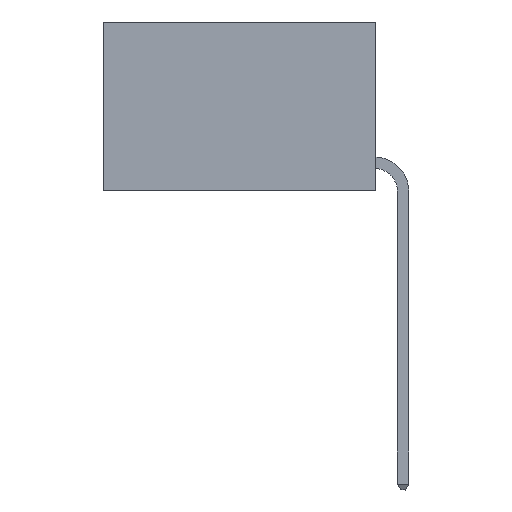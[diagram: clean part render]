
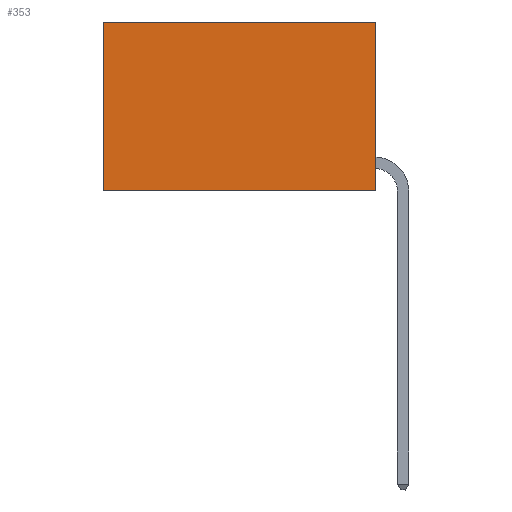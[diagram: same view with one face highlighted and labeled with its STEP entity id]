
A CAD part, left-side view. The second image highlights one B-rep face of the part: STEP entity #353.
In plain terms, the highlighted planar face has unit normal (-1, 0, 0).
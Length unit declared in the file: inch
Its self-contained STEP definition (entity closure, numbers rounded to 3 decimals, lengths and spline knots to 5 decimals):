
#353 = ADVANCED_FACE ( 'NONE', ( #5315 ), #7986, .F. ) ;
#680 = LINE ( 'NONE', #1629, #2735 ) ;
#691 = CARTESIAN_POINT ( 'NONE',  ( 0.2625, 0.6, -0.37 ) ) ;
#824 = VECTOR ( 'NONE', #7838, 39.37008 ) ;
#979 = EDGE_CURVE ( 'NONE', #7030, #5286, #6334, .T. ) ;
#1422 = CARTESIAN_POINT ( 'NONE',  ( 0.2625, 0., -0.37 ) ) ;
#1629 = CARTESIAN_POINT ( 'NONE',  ( 0.2625, 0., 0. ) ) ;
#1760 = EDGE_CURVE ( 'NONE', #7035, #7030, #680, .T. ) ;
#1838 = CARTESIAN_POINT ( 'NONE',  ( 0.2625, 0.6, 0. ) ) ;
#2067 = VECTOR ( 'NONE', #6882, 39.37008 ) ;
#2118 = LINE ( 'NONE', #5071, #8231 ) ;
#2173 = VERTEX_POINT ( 'NONE', #8725 ) ;
#2587 = DIRECTION ( 'NONE',  ( 0., 1., 0. ) ) ;
#2735 = VECTOR ( 'NONE', #2587, 39.37008 ) ;
#2865 = LINE ( 'NONE', #1422, #824 ) ;
#3281 = EDGE_LOOP ( 'NONE', ( #5196, #8546, #10106, #8673 ) ) ;
#3445 = DIRECTION ( 'NONE',  ( 0., 0., -1. ) ) ;
#4118 = EDGE_CURVE ( 'NONE', #7035, #2173, #2118, .T. ) ;
#4558 = CARTESIAN_POINT ( 'NONE',  ( 0.2625, 0., 0. ) ) ;
#5071 = CARTESIAN_POINT ( 'NONE',  ( 0.2625, 0., 0. ) ) ;
#5196 = ORIENTED_EDGE ( 'NONE', *, *, #979, .T. ) ;
#5286 = VERTEX_POINT ( 'NONE', #691 ) ;
#5315 = FACE_OUTER_BOUND ( 'NONE', #3281, .T. ) ;
#5656 = EDGE_CURVE ( 'NONE', #2173, #5286, #2865, .T. ) ;
#6306 = CARTESIAN_POINT ( 'NONE',  ( 0.2625, 0.6, 0. ) ) ;
#6334 = LINE ( 'NONE', #6306, #2067 ) ;
#6385 = AXIS2_PLACEMENT_3D ( 'NONE', #4558, #7142, #9906 ) ;
#6882 = DIRECTION ( 'NONE',  ( 0., 0., -1. ) ) ;
#7030 = VERTEX_POINT ( 'NONE', #1838 ) ;
#7035 = VERTEX_POINT ( 'NONE', #8216 ) ;
#7142 = DIRECTION ( 'NONE',  ( 1., 0., 0. ) ) ;
#7838 = DIRECTION ( 'NONE',  ( 0., 1., 0. ) ) ;
#7986 = PLANE ( 'NONE',  #6385 ) ;
#8216 = CARTESIAN_POINT ( 'NONE',  ( 0.2625, 0., 0. ) ) ;
#8231 = VECTOR ( 'NONE', #3445, 39.37008 ) ;
#8546 = ORIENTED_EDGE ( 'NONE', *, *, #5656, .F. ) ;
#8673 = ORIENTED_EDGE ( 'NONE', *, *, #1760, .T. ) ;
#8725 = CARTESIAN_POINT ( 'NONE',  ( 0.2625, 0., -0.37 ) ) ;
#9906 = DIRECTION ( 'NONE',  ( 0., 0., -1. ) ) ;
#10106 = ORIENTED_EDGE ( 'NONE', *, *, #4118, .F. ) ;
